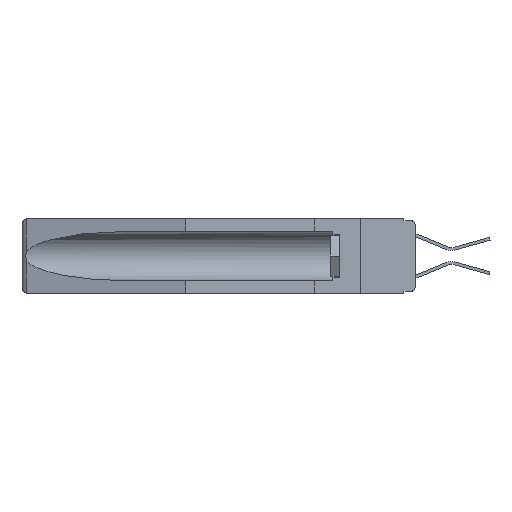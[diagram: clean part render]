
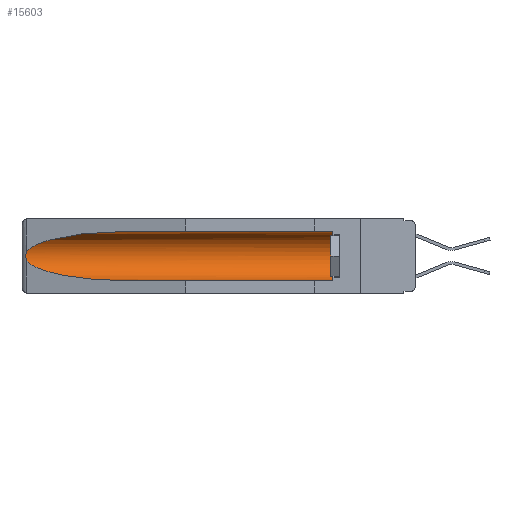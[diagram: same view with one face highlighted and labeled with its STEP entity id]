
A CAD part, left-side view. The second image highlights one B-rep face of the part: STEP entity #15603.
In plain terms, the highlighted cylindrical face has radius 2.857 mm (diameter 5.715 mm), a partial arc.
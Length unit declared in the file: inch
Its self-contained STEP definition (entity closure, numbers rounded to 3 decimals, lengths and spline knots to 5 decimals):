
#182 =( BOUNDED_CURVE ( )  B_SPLINE_CURVE ( 3, ( #15408, #11135, #15238, #15066 ),
 .UNSPECIFIED., .F., .F. ) 
 B_SPLINE_CURVE_WITH_KNOTS ( ( 4, 4 ),
 ( 4.71239, 6.08839 ),
 .UNSPECIFIED. ) 
 CURVE ( )  GEOMETRIC_REPRESENTATION_ITEM ( )  RATIONAL_B_SPLINE_CURVE ( ( 1., 0.848, 0.848, 1. ) ) 
 REPRESENTATION_ITEM ( '' )  );
#330 = DIRECTION ( 'NONE',  ( 0., 0., 1. ) ) ;
#355 = VECTOR ( 'NONE', #6530, 39.37008 ) ;
#654 = ORIENTED_EDGE ( 'NONE', *, *, #7664, .T. ) ;
#715 = CARTESIAN_POINT ( 'NONE',  ( 0.155, 1.07973, -0.059 ) ) ;
#892 = VERTEX_POINT ( 'NONE', #11525 ) ;
#1024 = CARTESIAN_POINT ( 'NONE',  ( 0.155, 0.126, -0.1715 ) ) ;
#1067 = CARTESIAN_POINT ( 'NONE',  ( 0.26655, 1.53094, -0.18657 ) ) ;
#1777 = ORIENTED_EDGE ( 'NONE', *, *, #6710, .T. ) ;
#1905 =( BOUNDED_CURVE ( )  B_SPLINE_CURVE ( 3, ( #11561, #13022, #9314, #10530 ),
 .UNSPECIFIED., .F., .F. ) 
 B_SPLINE_CURVE_WITH_KNOTS ( ( 4, 4 ),
 ( 0.1948, 1.5708 ),
 .UNSPECIFIED. ) 
 CURVE ( )  GEOMETRIC_REPRESENTATION_ITEM ( )  RATIONAL_B_SPLINE_CURVE ( ( 1., 0.848, 0.848, 1. ) ) 
 REPRESENTATION_ITEM ( '' )  );
#2451 = VERTEX_POINT ( 'NONE', #715 ) ;
#2468 = CARTESIAN_POINT ( 'NONE',  ( 0.155, 0.126, -0.059 ) ) ;
#2554 = LINE ( 'NONE', #7843, #355 ) ;
#3503 = CARTESIAN_POINT ( 'NONE',  ( 0.26537, 1.52718, -0.19328 ) ) ;
#3727 = CARTESIAN_POINT ( 'NONE',  ( 0.26597, 1.5296, -0.19026 ) ) ;
#4266 = CARTESIAN_POINT ( 'NONE',  ( 0.155, -0.30754, -0.1715 ) ) ;
#4756 = CARTESIAN_POINT ( 'NONE',  ( 0.26537, 1.52718, -0.19328 ) ) ;
#5638 = EDGE_CURVE ( 'NONE', #2451, #892, #182, .T. ) ;
#5907 = EDGE_CURVE ( 'NONE', #11881, #8771, #1905, .T. ) ;
#6156 = B_SPLINE_CURVE_WITH_KNOTS ( 'NONE', 3,
 ( #8987, #8809, #12518, #11229, #16780, #7382, #12853, #1067, #3727, #4756 ),
 .UNSPECIFIED., .F., .F.,
 ( 4, 2, 2, 2, 4 ),
 ( 0., 0.00029, 0.00058, 0.00087, 0.00117 ),
 .UNSPECIFIED. ) ;
#6530 = DIRECTION ( 'NONE',  ( 0., 1., 0. ) ) ;
#6543 = DIRECTION ( 'NONE',  ( 0., 0., 1. ) ) ;
#6710 = EDGE_CURVE ( 'NONE', #892, #11881, #6156, .T. ) ;
#6937 = DIRECTION ( 'NONE',  ( 0., 1., 0. ) ) ;
#6951 = EDGE_CURVE ( 'NONE', #11226, #8771, #12418, .T. ) ;
#7101 = ORIENTED_EDGE ( 'NONE', *, *, #9540, .T. ) ;
#7382 = CARTESIAN_POINT ( 'NONE',  ( 0.2675, 1.53308, -0.17534 ) ) ;
#7664 = EDGE_CURVE ( 'NONE', #11226, #16813, #13209, .T. ) ;
#7843 = CARTESIAN_POINT ( 'NONE',  ( 0.155, -0.30754, -0.059 ) ) ;
#8183 = AXIS2_PLACEMENT_3D ( 'NONE', #4266, #15704, #330 ) ;
#8771 = VERTEX_POINT ( 'NONE', #13512 ) ;
#8809 = CARTESIAN_POINT ( 'NONE',  ( 0.26597, 1.52961, -0.15275 ) ) ;
#8810 = ORIENTED_EDGE ( 'NONE', *, *, #6951, .F. ) ;
#8987 = CARTESIAN_POINT ( 'NONE',  ( 0.26537, 1.52718, -0.14972 ) ) ;
#9314 = CARTESIAN_POINT ( 'NONE',  ( 0.21114, 1.30732, -0.284 ) ) ;
#9521 = FACE_OUTER_BOUND ( 'NONE', #10384, .T. ) ;
#9540 = EDGE_CURVE ( 'NONE', #16813, #2451, #2554, .T. ) ;
#9657 = VECTOR ( 'NONE', #6937, 39.37008 ) ;
#10384 = EDGE_LOOP ( 'NONE', ( #10577, #1777, #11291, #8810, #654, #7101 ) ) ;
#10441 = CARTESIAN_POINT ( 'NONE',  ( 0.155, 0.126, -0.284 ) ) ;
#10530 = CARTESIAN_POINT ( 'NONE',  ( 0.155, 1.07973, -0.284 ) ) ;
#10577 = ORIENTED_EDGE ( 'NONE', *, *, #5638, .T. ) ;
#10583 = DIRECTION ( 'NONE',  ( 0., -1., 0. ) ) ;
#11135 = CARTESIAN_POINT ( 'NONE',  ( 0.21114, 1.30732, -0.059 ) ) ;
#11226 = VERTEX_POINT ( 'NONE', #10441 ) ;
#11229 = CARTESIAN_POINT ( 'NONE',  ( 0.2673, 1.5327, -0.16383 ) ) ;
#11291 = ORIENTED_EDGE ( 'NONE', *, *, #5907, .T. ) ;
#11525 = CARTESIAN_POINT ( 'NONE',  ( 0.26537, 1.52718, -0.14972 ) ) ;
#11561 = CARTESIAN_POINT ( 'NONE',  ( 0.26537, 1.52718, -0.19328 ) ) ;
#11881 = VERTEX_POINT ( 'NONE', #3503 ) ;
#12418 = LINE ( 'NONE', #13695, #9657 ) ;
#12518 = CARTESIAN_POINT ( 'NONE',  ( 0.26654, 1.53092, -0.15636 ) ) ;
#12853 = CARTESIAN_POINT ( 'NONE',  ( 0.2673, 1.53269, -0.17917 ) ) ;
#13022 = CARTESIAN_POINT ( 'NONE',  ( 0.25451, 1.48313, -0.24835 ) ) ;
#13209 = CIRCLE ( 'NONE', #16737, 0.1125 ) ;
#13512 = CARTESIAN_POINT ( 'NONE',  ( 0.155, 1.07973, -0.284 ) ) ;
#13695 = CARTESIAN_POINT ( 'NONE',  ( 0.155, -0.30754, -0.284 ) ) ;
#14678 = CYLINDRICAL_SURFACE ( 'NONE', #8183, 0.1125 ) ;
#15066 = CARTESIAN_POINT ( 'NONE',  ( 0.26537, 1.52718, -0.14972 ) ) ;
#15238 = CARTESIAN_POINT ( 'NONE',  ( 0.25451, 1.48313, -0.09465 ) ) ;
#15408 = CARTESIAN_POINT ( 'NONE',  ( 0.155, 1.07973, -0.059 ) ) ;
#15603 = ADVANCED_FACE ( 'NONE', ( #9521 ), #14678, .F. ) ;
#15704 = DIRECTION ( 'NONE',  ( 0., 1., 0. ) ) ;
#16737 = AXIS2_PLACEMENT_3D ( 'NONE', #1024, #10583, #6543 ) ;
#16780 = CARTESIAN_POINT ( 'NONE',  ( 0.2675, 1.53308, -0.16763 ) ) ;
#16813 = VERTEX_POINT ( 'NONE', #2468 ) ;
